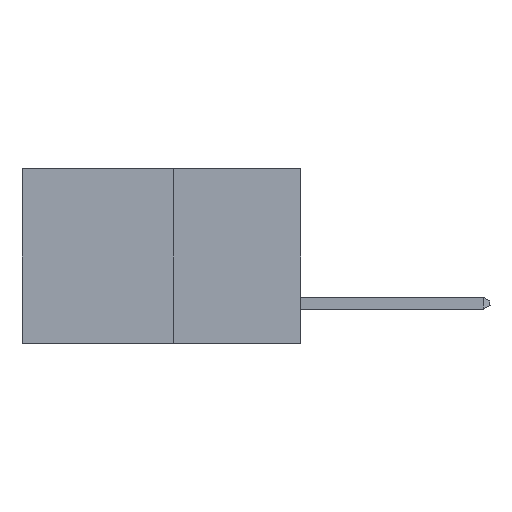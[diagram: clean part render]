
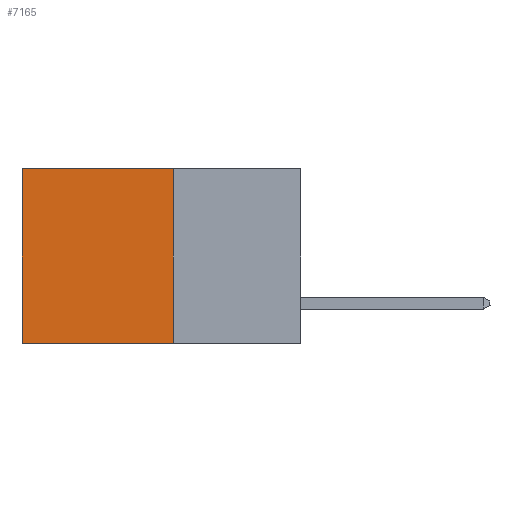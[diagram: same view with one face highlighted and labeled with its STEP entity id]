
A CAD part, left-side view. The second image highlights one B-rep face of the part: STEP entity #7165.
In plain terms, the highlighted planar face has unit normal (-1, 0, 0).
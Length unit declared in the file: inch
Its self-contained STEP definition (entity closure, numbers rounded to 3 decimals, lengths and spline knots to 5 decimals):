
#268 = LINE ( 'NONE', #32497, #24168 ) ;
#2766 = CARTESIAN_POINT ( 'NONE',  ( 0.277, 0.27, 0. ) ) ;
#2812 = CARTESIAN_POINT ( 'NONE',  ( 0.277, 0.59, -0.37 ) ) ;
#2894 = CARTESIAN_POINT ( 'NONE',  ( 0.277, 0.27, -0.37 ) ) ;
#2986 = LINE ( 'NONE', #6914, #10120 ) ;
#5237 = FACE_OUTER_BOUND ( 'NONE', #24824, .T. ) ;
#6118 = CARTESIAN_POINT ( 'NONE',  ( 0.277, 0.59, 0. ) ) ;
#6914 = CARTESIAN_POINT ( 'NONE',  ( 0.277, 0.27, -0.37 ) ) ;
#7099 = AXIS2_PLACEMENT_3D ( 'NONE', #22996, #22950, #22904 ) ;
#7165 = ADVANCED_FACE ( 'NONE', ( #5237 ), #23249, .F. ) ;
#8522 = VERTEX_POINT ( 'NONE', #2812 ) ;
#9873 = DIRECTION ( 'NONE',  ( 0., 0., -1. ) ) ;
#10120 = VECTOR ( 'NONE', #24687, 39.37008 ) ;
#13991 = VERTEX_POINT ( 'NONE', #2894 ) ;
#14159 = VERTEX_POINT ( 'NONE', #6118 ) ;
#14328 = VERTEX_POINT ( 'NONE', #31855 ) ;
#14961 = ORIENTED_EDGE ( 'NONE', *, *, #26051, .T. ) ;
#16720 = ORIENTED_EDGE ( 'NONE', *, *, #28876, .F. ) ;
#20135 = ORIENTED_EDGE ( 'NONE', *, *, #26937, .F. ) ;
#20910 = VECTOR ( 'NONE', #25655, 39.37008 ) ;
#21332 = CARTESIAN_POINT ( 'NONE',  ( 0.277, 0.59, -0.37 ) ) ;
#21764 = ORIENTED_EDGE ( 'NONE', *, *, #24449, .T. ) ;
#22904 = DIRECTION ( 'NONE',  ( 0., 0., -1. ) ) ;
#22950 = DIRECTION ( 'NONE',  ( 1., 0., 0. ) ) ;
#22996 = CARTESIAN_POINT ( 'NONE',  ( 0.277, 0.27, -0.37 ) ) ;
#23249 = PLANE ( 'NONE',  #7099 ) ;
#23916 = DIRECTION ( 'NONE',  ( 0., 0., -1. ) ) ;
#24168 = VECTOR ( 'NONE', #9873, 39.37008 ) ;
#24449 = EDGE_CURVE ( 'NONE', #14328, #14159, #26884, .T. ) ;
#24687 = DIRECTION ( 'NONE',  ( 0., 1., 0. ) ) ;
#24824 = EDGE_LOOP ( 'NONE', ( #14961, #16720, #20135, #21764 ) ) ;
#25655 = DIRECTION ( 'NONE',  ( 0., 1., 0. ) ) ;
#25811 = VECTOR ( 'NONE', #23916, 39.37008 ) ;
#26051 = EDGE_CURVE ( 'NONE', #14159, #8522, #27381, .T. ) ;
#26884 = LINE ( 'NONE', #2766, #20910 ) ;
#26937 = EDGE_CURVE ( 'NONE', #14328, #13991, #268, .T. ) ;
#27381 = LINE ( 'NONE', #21332, #25811 ) ;
#28876 = EDGE_CURVE ( 'NONE', #13991, #8522, #2986, .T. ) ;
#31855 = CARTESIAN_POINT ( 'NONE',  ( 0.277, 0.27, 0. ) ) ;
#32497 = CARTESIAN_POINT ( 'NONE',  ( 0.277, 0.27, -0.37 ) ) ;
